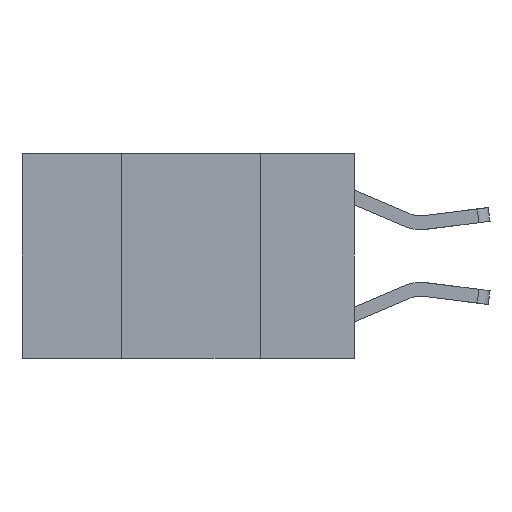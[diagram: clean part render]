
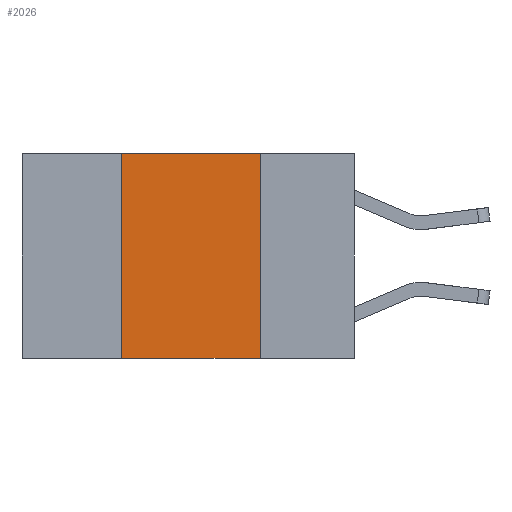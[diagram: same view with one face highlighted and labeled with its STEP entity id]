
A CAD part, left-side view. The second image highlights one B-rep face of the part: STEP entity #2026.
In plain terms, the highlighted planar face has unit normal (-1, 0, 0).
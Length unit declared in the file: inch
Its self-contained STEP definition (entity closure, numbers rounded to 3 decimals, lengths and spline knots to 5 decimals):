
#214 = CARTESIAN_POINT ( 'NONE',  ( 0., 0.17, 0. ) ) ;
#238 = DIRECTION ( 'NONE',  ( 0., 0., -1. ) ) ;
#840 = DIRECTION ( 'NONE',  ( 0., -1., 0. ) ) ;
#897 = VECTOR ( 'NONE', #8373, 39.37008 ) ;
#962 = ORIENTED_EDGE ( 'NONE', *, *, #4286, .F. ) ;
#966 = CARTESIAN_POINT ( 'NONE',  ( 0., 0.6, 0. ) ) ;
#1006 = LINE ( 'NONE', #8246, #897 ) ;
#1033 = EDGE_LOOP ( 'NONE', ( #8930, #962, #9509, #3719 ) ) ;
#1154 = VECTOR ( 'NONE', #4594, 39.37008 ) ;
#1336 = EDGE_CURVE ( 'NONE', #5586, #10889, #7124, .T. ) ;
#1408 = LINE ( 'NONE', #6860, #9275 ) ;
#1894 = DIRECTION ( 'NONE',  ( 1., 0., 0. ) ) ;
#2026 = ADVANCED_FACE ( 'NONE', ( #11036 ), #2884, .F. ) ;
#2771 = CARTESIAN_POINT ( 'NONE',  ( 0., 0.6, 0. ) ) ;
#2884 = PLANE ( 'NONE',  #6780 ) ;
#3654 = CARTESIAN_POINT ( 'NONE',  ( 0., 0.42, -0.37 ) ) ;
#3719 = ORIENTED_EDGE ( 'NONE', *, *, #1336, .T. ) ;
#3720 = VECTOR ( 'NONE', #840, 39.37008 ) ;
#4286 = EDGE_CURVE ( 'NONE', #5200, #5631, #9111, .T. ) ;
#4594 = DIRECTION ( 'NONE',  ( 0., -1., 0. ) ) ;
#5200 = VERTEX_POINT ( 'NONE', #9503 ) ;
#5586 = VERTEX_POINT ( 'NONE', #3654 ) ;
#5631 = VERTEX_POINT ( 'NONE', #214 ) ;
#6191 = CARTESIAN_POINT ( 'NONE',  ( 0., 0.6, -0.37 ) ) ;
#6780 = AXIS2_PLACEMENT_3D ( 'NONE', #2771, #1894, #238 ) ;
#6860 = CARTESIAN_POINT ( 'NONE',  ( 0., 0.17, 0. ) ) ;
#7124 = LINE ( 'NONE', #6191, #3720 ) ;
#8246 = CARTESIAN_POINT ( 'NONE',  ( 0., 0.42, 0. ) ) ;
#8373 = DIRECTION ( 'NONE',  ( 0., 0., 1. ) ) ;
#8930 = ORIENTED_EDGE ( 'NONE', *, *, #10443, .F. ) ;
#9111 = LINE ( 'NONE', #966, #1154 ) ;
#9275 = VECTOR ( 'NONE', #9724, 39.37008 ) ;
#9503 = CARTESIAN_POINT ( 'NONE',  ( 0., 0.42, 0. ) ) ;
#9509 = ORIENTED_EDGE ( 'NONE', *, *, #9995, .F. ) ;
#9724 = DIRECTION ( 'NONE',  ( 0., 0., -1. ) ) ;
#9995 = EDGE_CURVE ( 'NONE', #5586, #5200, #1006, .T. ) ;
#10443 = EDGE_CURVE ( 'NONE', #5631, #10889, #1408, .T. ) ;
#10889 = VERTEX_POINT ( 'NONE', #11370 ) ;
#11036 = FACE_OUTER_BOUND ( 'NONE', #1033, .T. ) ;
#11370 = CARTESIAN_POINT ( 'NONE',  ( 0., 0.17, -0.37 ) ) ;
